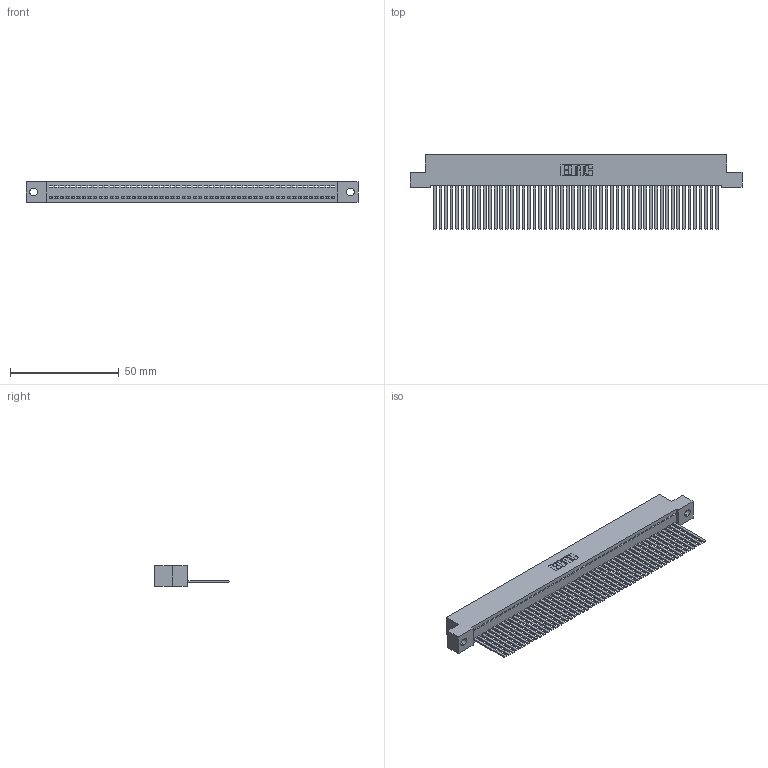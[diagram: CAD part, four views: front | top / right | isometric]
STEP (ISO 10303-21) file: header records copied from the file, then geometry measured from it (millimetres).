
FILE_DESCRIPTION (( 'STEP AP203' ), '1' );
FILE_NAME ('342-052-544-102.STEP', '2018-08-12T22:14:57', ( '' ), ( '' ), 'SwSTEP 2.0', 'SolidWorks 2016', '' );
FILE_SCHEMA (( 'CONFIG_CONTROL_DESIGN' ));
Length unit declared in the file: inch
Products named in the file (3): 342 Part_.128 Slot; 345-292-001_345-293-144; 342-052-544-102
Assembly tree (53 placements, depth 2):
  342-052-544-102
    342 Part_.128 Slot
    345-292-001_345-293-144  x52
Bounding box: 152.4 x 34.3 x 9.4 mm (x, y, z)
Volume: 13949.3 mm3; surface area: 22144.3 mm2
Topology: 53 solids, 53 shells, 2818 faces, 8527 edges, 5614 vertices
Faces by surface type: plane 2046, cylinder 772
Entity records: 30315 total; most frequent: CARTESIAN_POINT 5234, ORIENTED_EDGE 5222, DIRECTION 4391, EDGE_CURVE 2611, VECTOR 2487, LINE 2487, VERTEX_POINT 1738, AXIS2_PLACEMENT_3D 952
